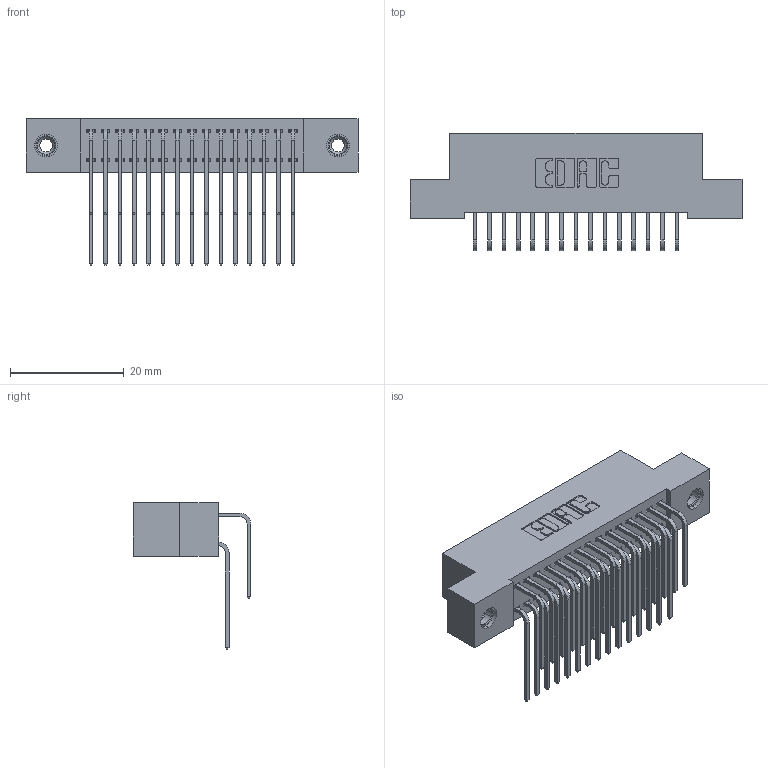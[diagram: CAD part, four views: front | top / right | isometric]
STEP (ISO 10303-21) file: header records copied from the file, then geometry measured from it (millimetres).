
FILE_DESCRIPTION (( 'STEP AP203' ), '1' );
FILE_NAME ('342-030-559-208.STEP', '2019-10-02T05:14:06', ( '' ), ( '' ), 'SwSTEP 2.0', 'SolidWorks 2016', '' );
FILE_SCHEMA (( 'CONFIG_CONTROL_DESIGN' ));
Length unit declared in the file: inch
Products named in the file (5): 342 Part_TI; 345-292-001_558 559 Tail - 1; 345-292-001_559 Tail - 2; 345-250-001_345-250-003-102; 342-030-559-208
Assembly tree (33 placements, depth 2):
  342-030-559-208
    342 Part_TI
    345-292-001_558 559 Tail - 1  x15
    345-292-001_559 Tail - 2  x15
    345-250-001_345-250-003-102  x2
Bounding box: 58.42 x 20.64 x 25.78 mm (x, y, z)
Volume: 5288.6 mm3; surface area: 8736.4 mm2
Topology: 33 solids, 33 shells, 1790 faces, 5265 edges, 3462 vertices
Faces by surface type: plane 1238, cylinder 536, cone 12, torus 4
Entity records: 15980 total; most frequent: CARTESIAN_POINT 2712, ORIENTED_EDGE 2590, DIRECTION 2377, EDGE_CURVE 1295, LINE 1107, VECTOR 1107, VERTEX_POINT 856, AXIS2_PLACEMENT_3D 635
